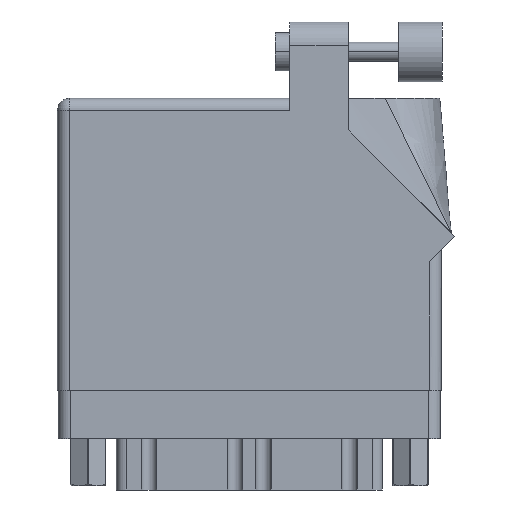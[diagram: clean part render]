
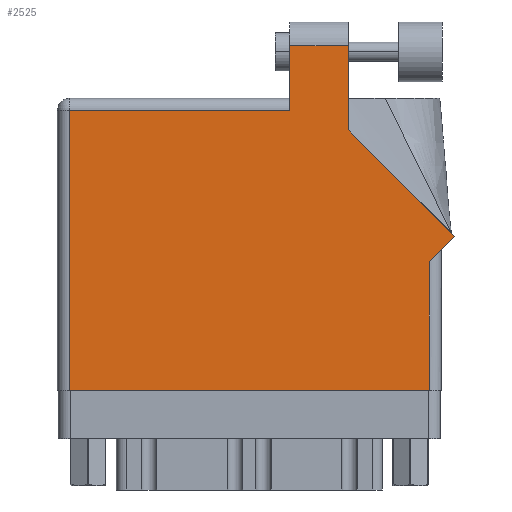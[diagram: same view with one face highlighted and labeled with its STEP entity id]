
A CAD part, front view. The second image highlights one B-rep face of the part: STEP entity #2525.
In plain terms, the highlighted face is planar.
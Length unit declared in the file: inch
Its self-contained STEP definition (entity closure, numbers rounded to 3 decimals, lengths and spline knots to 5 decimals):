
#480 = VECTOR ( 'NONE', #37525, 39.37008 ) ;
#1712 = CARTESIAN_POINT ( 'NONE',  ( 0.062, 0., 0. ) ) ;
#2275 = CARTESIAN_POINT ( 'NONE',  ( 1.948, 0.737, 0. ) ) ;
#2525 = ADVANCED_FACE ( 'NONE', ( #46084 ), #23296, .F. ) ;
#2943 = LINE ( 'NONE', #39637, #17402 ) ;
#3563 = CARTESIAN_POINT ( 'NONE',  ( 1.948, 0.675, 0. ) ) ;
#4816 = CARTESIAN_POINT ( 'NONE',  ( 1.217, 1.53, 0. ) ) ;
#4852 = EDGE_CURVE ( 'NONE', #34883, #37979, #2943, .T. ) ;
#5229 = VECTOR ( 'NONE', #13963, 39.37008 ) ;
#5503 = VERTEX_POINT ( 'NONE', #33324 ) ;
#9626 = CARTESIAN_POINT ( 'NONE',  ( 0., 1.53, 0. ) ) ;
#9838 = VECTOR ( 'NONE', #43429, 39.37008 ) ;
#12454 = EDGE_LOOP ( 'NONE', ( #35329, #33420, #39633, #32108, #39041, #37226, #26896, #32819, #19067 ) ) ;
#12820 = EDGE_CURVE ( 'NONE', #14763, #20045, #23292, .T. ) ;
#12974 = EDGE_CURVE ( 'NONE', #19007, #38500, #12976, .T. ) ;
#12976 = LINE ( 'NONE', #19703, #17117 ) ;
#13467 = DIRECTION ( 'NONE',  ( 0., 0., -1. ) ) ;
#13963 = DIRECTION ( 'NONE',  ( -1., 0., 0. ) ) ;
#14317 = EDGE_CURVE ( 'NONE', #38500, #14763, #41853, .T. ) ;
#14763 = VERTEX_POINT ( 'NONE', #1712 ) ;
#15183 = DIRECTION ( 'NONE',  ( 1., 0., 0. ) ) ;
#15403 = CARTESIAN_POINT ( 'NONE',  ( 1.217, 1.468, 0. ) ) ;
#15633 = DIRECTION ( 'NONE',  ( 0., -1., 0. ) ) ;
#17117 = VECTOR ( 'NONE', #27361, 39.37008 ) ;
#17220 = EDGE_CURVE ( 'NONE', #20045, #41009, #24116, .T. ) ;
#17402 = VECTOR ( 'NONE', #25242, 39.37008 ) ;
#17535 = EDGE_CURVE ( 'NONE', #36646, #19007, #27360, .T. ) ;
#17985 = EDGE_CURVE ( 'NONE', #41009, #5503, #40512, .T. ) ;
#19007 = VERTEX_POINT ( 'NONE', #15403 ) ;
#19019 = CARTESIAN_POINT ( 'NONE',  ( 2.08071, 0.80771, 0. ) ) ;
#19067 = ORIENTED_EDGE ( 'NONE', *, *, #38020, .T. ) ;
#19250 = LINE ( 'NONE', #19019, #23559 ) ;
#19703 = CARTESIAN_POINT ( 'NONE',  ( 0., 1.468, 0. ) ) ;
#20045 = VERTEX_POINT ( 'NONE', #27428 ) ;
#20876 = DIRECTION ( 'NONE',  ( -1., 0., 0. ) ) ;
#21631 = CARTESIAN_POINT ( 'NONE',  ( 1.524, 1.36442, 0. ) ) ;
#22677 = VECTOR ( 'NONE', #15183, 39.37008 ) ;
#23292 = LINE ( 'NONE', #25959, #22677 ) ;
#23296 = PLANE ( 'NONE',  #39251 ) ;
#23559 = VECTOR ( 'NONE', #45152, 39.37008 ) ;
#24116 = LINE ( 'NONE', #2275, #28660 ) ;
#24745 = CARTESIAN_POINT ( 'NONE',  ( 1.217, 1.805, 0. ) ) ;
#25242 = DIRECTION ( 'NONE',  ( 0., 1., 0. ) ) ;
#25959 = CARTESIAN_POINT ( 'NONE',  ( 0., 0., 0. ) ) ;
#26263 = CARTESIAN_POINT ( 'NONE',  ( 0.062, 1.468, 0. ) ) ;
#26732 = CARTESIAN_POINT ( 'NONE',  ( 0.062, 0., 0. ) ) ;
#26896 = ORIENTED_EDGE ( 'NONE', *, *, #17220, .T. ) ;
#27360 = LINE ( 'NONE', #4816, #34018 ) ;
#27361 = DIRECTION ( 'NONE',  ( -1., 0., 0. ) ) ;
#27428 = CARTESIAN_POINT ( 'NONE',  ( 1.948, 0., 0. ) ) ;
#28660 = VECTOR ( 'NONE', #31547, 39.37008 ) ;
#29040 = LINE ( 'NONE', #24745, #5229 ) ;
#31547 = DIRECTION ( 'NONE',  ( 0., 1., 0. ) ) ;
#32108 = ORIENTED_EDGE ( 'NONE', *, *, #12974, .T. ) ;
#32819 = ORIENTED_EDGE ( 'NONE', *, *, #17985, .T. ) ;
#33324 = CARTESIAN_POINT ( 'NONE',  ( 2.08071, 0.80771, 0. ) ) ;
#33420 = ORIENTED_EDGE ( 'NONE', *, *, #39160, .T. ) ;
#34018 = VECTOR ( 'NONE', #15633, 39.37008 ) ;
#34883 = VERTEX_POINT ( 'NONE', #21631 ) ;
#35329 = ORIENTED_EDGE ( 'NONE', *, *, #4852, .T. ) ;
#36646 = VERTEX_POINT ( 'NONE', #41679 ) ;
#37226 = ORIENTED_EDGE ( 'NONE', *, *, #12820, .T. ) ;
#37464 = CARTESIAN_POINT ( 'NONE',  ( 1.524, 1.805, 0. ) ) ;
#37525 = DIRECTION ( 'NONE',  ( 0., -1., 0. ) ) ;
#37979 = VERTEX_POINT ( 'NONE', #37464 ) ;
#38020 = EDGE_CURVE ( 'NONE', #5503, #34883, #19250, .T. ) ;
#38500 = VERTEX_POINT ( 'NONE', #26263 ) ;
#39041 = ORIENTED_EDGE ( 'NONE', *, *, #14317, .T. ) ;
#39160 = EDGE_CURVE ( 'NONE', #37979, #36646, #29040, .T. ) ;
#39251 = AXIS2_PLACEMENT_3D ( 'NONE', #9626, #13467, #20876 ) ;
#39633 = ORIENTED_EDGE ( 'NONE', *, *, #17535, .T. ) ;
#39637 = CARTESIAN_POINT ( 'NONE',  ( 1.524, 1.36442, 0. ) ) ;
#40290 = CARTESIAN_POINT ( 'NONE',  ( 2.01, 0.737, 0. ) ) ;
#40512 = LINE ( 'NONE', #40290, #9838 ) ;
#41009 = VERTEX_POINT ( 'NONE', #3563 ) ;
#41679 = CARTESIAN_POINT ( 'NONE',  ( 1.217, 1.805, 0. ) ) ;
#41853 = LINE ( 'NONE', #26732, #480 ) ;
#43429 = DIRECTION ( 'NONE',  ( 0.707, 0.707, 0. ) ) ;
#45152 = DIRECTION ( 'NONE',  ( -0.707, 0.707, 0. ) ) ;
#46084 = FACE_OUTER_BOUND ( 'NONE', #12454, .T. ) ;
